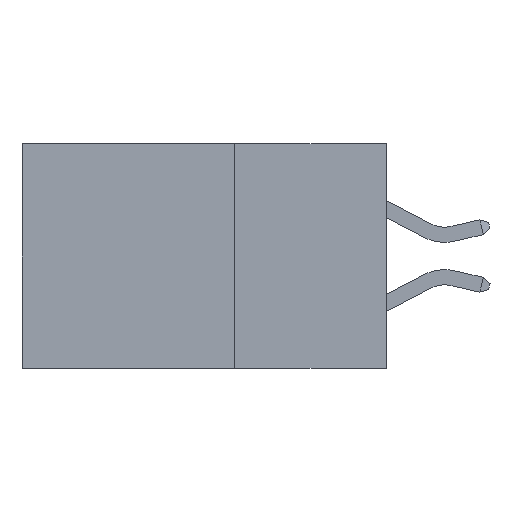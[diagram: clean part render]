
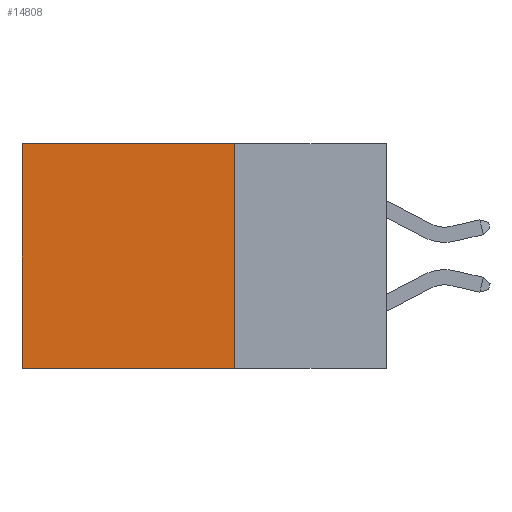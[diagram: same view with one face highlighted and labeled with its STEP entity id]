
A CAD part, left-side view. The second image highlights one B-rep face of the part: STEP entity #14808.
In plain terms, the highlighted planar face has unit normal (-1, 0, 0).
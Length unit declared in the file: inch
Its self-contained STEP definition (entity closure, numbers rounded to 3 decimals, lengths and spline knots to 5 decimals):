
#167 = LINE ( 'NONE', #13008, #15673 ) ;
#244 = LINE ( 'NONE', #8395, #24976 ) ;
#714 = CARTESIAN_POINT ( 'NONE',  ( 0.2615, 0.25, -0.37 ) ) ;
#986 = ORIENTED_EDGE ( 'NONE', *, *, #15950, .T. ) ;
#1415 = PLANE ( 'NONE',  #4377 ) ;
#3427 = DIRECTION ( 'NONE',  ( 1., 0., 0. ) ) ;
#3904 = EDGE_LOOP ( 'NONE', ( #6215, #4931, #17758, #986 ) ) ;
#4377 = AXIS2_PLACEMENT_3D ( 'NONE', #13507, #3427, #17528 ) ;
#4931 = ORIENTED_EDGE ( 'NONE', *, *, #20801, .F. ) ;
#6027 = LINE ( 'NONE', #714, #11428 ) ;
#6215 = ORIENTED_EDGE ( 'NONE', *, *, #22924, .T. ) ;
#6425 = CARTESIAN_POINT ( 'NONE',  ( 0.2615, 0.6, 0. ) ) ;
#7169 = CARTESIAN_POINT ( 'NONE',  ( 0.2615, 0.6, -0.37 ) ) ;
#7547 = VERTEX_POINT ( 'NONE', #13937 ) ;
#8395 = CARTESIAN_POINT ( 'NONE',  ( 0.2615, 0.25, -0.37 ) ) ;
#8903 = DIRECTION ( 'NONE',  ( 0., 1., 0. ) ) ;
#9232 = DIRECTION ( 'NONE',  ( 0., 0., -1. ) ) ;
#10445 = FACE_OUTER_BOUND ( 'NONE', #3904, .T. ) ;
#10831 = LINE ( 'NONE', #7169, #20811 ) ;
#11428 = VECTOR ( 'NONE', #20716, 39.37008 ) ;
#13008 = CARTESIAN_POINT ( 'NONE',  ( 0.2615, 0.25, 0. ) ) ;
#13052 = VERTEX_POINT ( 'NONE', #18452 ) ;
#13507 = CARTESIAN_POINT ( 'NONE',  ( 0.2615, 0.25, -0.37 ) ) ;
#13849 = EDGE_CURVE ( 'NONE', #7547, #24053, #6027, .T. ) ;
#13937 = CARTESIAN_POINT ( 'NONE',  ( 0.2615, 0.25, 0. ) ) ;
#14808 = ADVANCED_FACE ( 'NONE', ( #10445 ), #1415, .F. ) ;
#15673 = VECTOR ( 'NONE', #8903, 39.37008 ) ;
#15950 = EDGE_CURVE ( 'NONE', #7547, #18931, #167, .T. ) ;
#17528 = DIRECTION ( 'NONE',  ( 0., 0., -1. ) ) ;
#17758 = ORIENTED_EDGE ( 'NONE', *, *, #13849, .F. ) ;
#18452 = CARTESIAN_POINT ( 'NONE',  ( 0.2615, 0.6, -0.37 ) ) ;
#18931 = VERTEX_POINT ( 'NONE', #6425 ) ;
#20716 = DIRECTION ( 'NONE',  ( 0., 0., -1. ) ) ;
#20801 = EDGE_CURVE ( 'NONE', #24053, #13052, #244, .T. ) ;
#20811 = VECTOR ( 'NONE', #9232, 39.37008 ) ;
#22924 = EDGE_CURVE ( 'NONE', #18931, #13052, #10831, .T. ) ;
#24053 = VERTEX_POINT ( 'NONE', #24340 ) ;
#24340 = CARTESIAN_POINT ( 'NONE',  ( 0.2615, 0.25, -0.37 ) ) ;
#24350 = DIRECTION ( 'NONE',  ( 0., 1., 0. ) ) ;
#24976 = VECTOR ( 'NONE', #24350, 39.37008 ) ;
